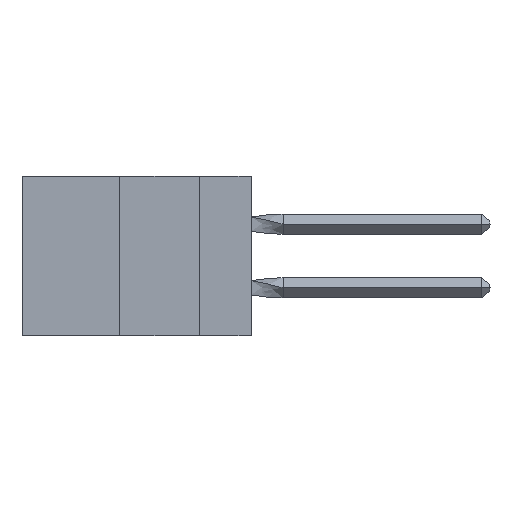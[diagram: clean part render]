
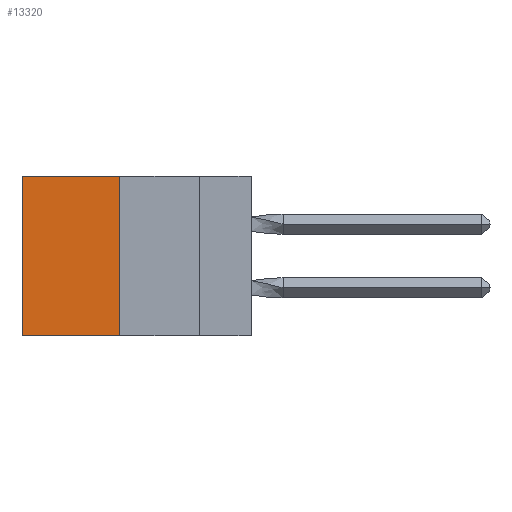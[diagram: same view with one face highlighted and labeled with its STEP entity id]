
A CAD part, left-side view. The second image highlights one B-rep face of the part: STEP entity #13320.
In plain terms, the highlighted planar face has unit normal (-1, 0, 0).
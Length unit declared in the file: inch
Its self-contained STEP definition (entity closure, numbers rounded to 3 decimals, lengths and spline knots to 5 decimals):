
#59 = VERTEX_POINT ( 'NONE', #13488 ) ;
#88 = CARTESIAN_POINT ( 'NONE',  ( 0.305, 0.413, -0.5 ) ) ;
#1238 = VERTEX_POINT ( 'NONE', #8051 ) ;
#1478 = ORIENTED_EDGE ( 'NONE', *, *, #10929, .T. ) ;
#2209 = DIRECTION ( 'NONE',  ( 0., 1., 0. ) ) ;
#2540 = LINE ( 'NONE', #88, #5339 ) ;
#3494 = LINE ( 'NONE', #8216, #8916 ) ;
#3620 = DIRECTION ( 'NONE',  ( 0., 0., -1. ) ) ;
#3667 = ORIENTED_EDGE ( 'NONE', *, *, #11043, .F. ) ;
#4167 = VECTOR ( 'NONE', #7757, 39.37008 ) ;
#4225 = EDGE_CURVE ( 'NONE', #10259, #4359, #8943, .T. ) ;
#4359 = VERTEX_POINT ( 'NONE', #9040 ) ;
#4977 = LINE ( 'NONE', #5741, #7437 ) ;
#5162 = FACE_OUTER_BOUND ( 'NONE', #9945, .T. ) ;
#5339 = VECTOR ( 'NONE', #2209, 39.37008 ) ;
#5675 = AXIS2_PLACEMENT_3D ( 'NONE', #12096, #8905, #3620 ) ;
#5696 = CARTESIAN_POINT ( 'NONE',  ( 0.305, 0.72, -0.5 ) ) ;
#5741 = CARTESIAN_POINT ( 'NONE',  ( 0.305, 0.413, 0. ) ) ;
#6751 = CARTESIAN_POINT ( 'NONE',  ( 0.305, 0.72, 0. ) ) ;
#6918 = ORIENTED_EDGE ( 'NONE', *, *, #8858, .F. ) ;
#7051 = DIRECTION ( 'NONE',  ( 0., 0., -1. ) ) ;
#7437 = VECTOR ( 'NONE', #10079, 39.37008 ) ;
#7757 = DIRECTION ( 'NONE',  ( 0., 0., -1. ) ) ;
#8051 = CARTESIAN_POINT ( 'NONE',  ( 0.305, 0.413, -0.5 ) ) ;
#8216 = CARTESIAN_POINT ( 'NONE',  ( 0.305, 0.413, -0.5 ) ) ;
#8858 = EDGE_CURVE ( 'NONE', #1238, #4359, #2540, .T. ) ;
#8905 = DIRECTION ( 'NONE',  ( 1., 0., 0. ) ) ;
#8916 = VECTOR ( 'NONE', #7051, 39.37008 ) ;
#8943 = LINE ( 'NONE', #5696, #4167 ) ;
#9040 = CARTESIAN_POINT ( 'NONE',  ( 0.305, 0.72, -0.5 ) ) ;
#9945 = EDGE_LOOP ( 'NONE', ( #11030, #6918, #3667, #1478 ) ) ;
#10079 = DIRECTION ( 'NONE',  ( 0., 1., 0. ) ) ;
#10259 = VERTEX_POINT ( 'NONE', #6751 ) ;
#10929 = EDGE_CURVE ( 'NONE', #59, #10259, #4977, .T. ) ;
#11030 = ORIENTED_EDGE ( 'NONE', *, *, #4225, .T. ) ;
#11043 = EDGE_CURVE ( 'NONE', #59, #1238, #3494, .T. ) ;
#12096 = CARTESIAN_POINT ( 'NONE',  ( 0.305, 0.413, -0.5 ) ) ;
#13081 = PLANE ( 'NONE',  #5675 ) ;
#13320 = ADVANCED_FACE ( 'NONE', ( #5162 ), #13081, .F. ) ;
#13488 = CARTESIAN_POINT ( 'NONE',  ( 0.305, 0.413, 0. ) ) ;
